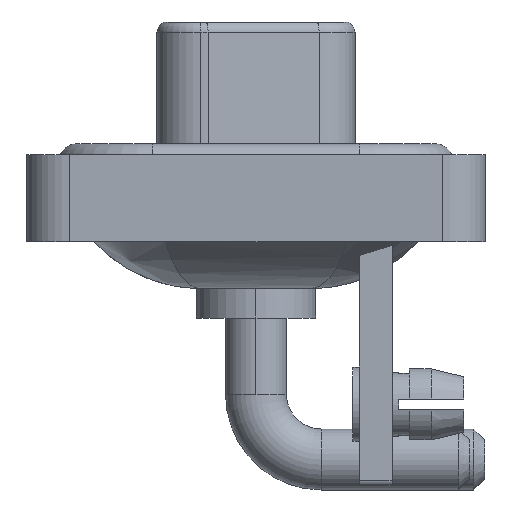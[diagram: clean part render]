
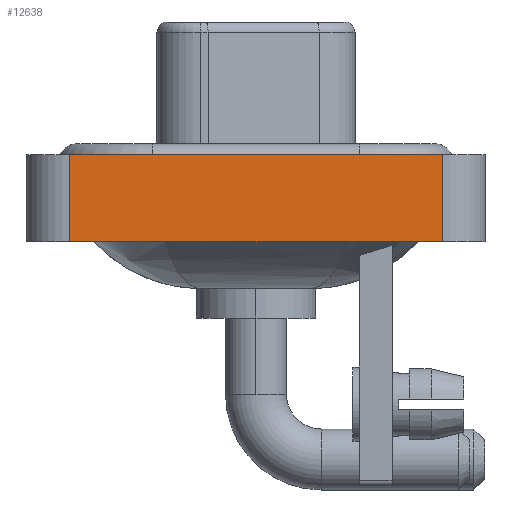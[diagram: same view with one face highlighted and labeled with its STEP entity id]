
A CAD part, left-side view. The second image highlights one B-rep face of the part: STEP entity #12638.
In plain terms, the highlighted planar face has unit normal (-1, 0, 0).
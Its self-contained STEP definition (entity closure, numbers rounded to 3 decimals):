
#395 = ORIENTED_EDGE ( 'NONE', *, *, #15056, .T. ) ;
#424 = DIRECTION ( 'NONE',  ( -1., 0., 0. ) ) ;
#551 = EDGE_CURVE ( 'NONE', #1799, #4549, #3963, .T. ) ;
#833 = CARTESIAN_POINT ( 'NONE',  ( -7.3, -8.55, -3.6 ) ) ;
#1799 = VERTEX_POINT ( 'NONE', #8385 ) ;
#2810 = LINE ( 'NONE', #7864, #3487 ) ;
#3487 = VECTOR ( 'NONE', #6222, 1000. ) ;
#3963 = LINE ( 'NONE', #5728, #11612 ) ;
#4293 = CARTESIAN_POINT ( 'NONE',  ( -7.3, -8.55, 0.4 ) ) ;
#4380 = ORIENTED_EDGE ( 'NONE', *, *, #19439, .T. ) ;
#4383 = VERTEX_POINT ( 'NONE', #833 ) ;
#4549 = VERTEX_POINT ( 'NONE', #11537 ) ;
#4615 = ORIENTED_EDGE ( 'NONE', *, *, #5329, .F. ) ;
#5329 = EDGE_CURVE ( 'NONE', #4549, #21401, #7590, .T. ) ;
#5728 = CARTESIAN_POINT ( 'NONE',  ( -7.3, 8.55, -3.6 ) ) ;
#5864 = DIRECTION ( 'NONE',  ( 0., -1., 0. ) ) ;
#6222 = DIRECTION ( 'NONE',  ( 0., 0., 1. ) ) ;
#7126 = DIRECTION ( 'NONE',  ( 0., 0., 1. ) ) ;
#7590 = LINE ( 'NONE', #4293, #11551 ) ;
#7609 = ORIENTED_EDGE ( 'NONE', *, *, #551, .F. ) ;
#7864 = CARTESIAN_POINT ( 'NONE',  ( -7.3, -8.55, -3.6 ) ) ;
#8385 = CARTESIAN_POINT ( 'NONE',  ( -7.3, 8.55, -3.6 ) ) ;
#9410 = CARTESIAN_POINT ( 'NONE',  ( -7.3, -8.55, 0.4 ) ) ;
#10399 = FACE_OUTER_BOUND ( 'NONE', #15369, .T. ) ;
#10865 = LINE ( 'NONE', #14273, #20759 ) ;
#11537 = CARTESIAN_POINT ( 'NONE',  ( -7.3, 8.55, 0.4 ) ) ;
#11551 = VECTOR ( 'NONE', #12483, 1000. ) ;
#11612 = VECTOR ( 'NONE', #16824, 1000. ) ;
#12483 = DIRECTION ( 'NONE',  ( 0., -1., 0. ) ) ;
#12638 = ADVANCED_FACE ( 'NONE', ( #10399 ), #13670, .T. ) ;
#13442 = AXIS2_PLACEMENT_3D ( 'NONE', #17101, #424, #7126 ) ;
#13670 = PLANE ( 'NONE',  #13442 ) ;
#14273 = CARTESIAN_POINT ( 'NONE',  ( -7.3, -8.55, -3.6 ) ) ;
#15056 = EDGE_CURVE ( 'NONE', #1799, #4383, #10865, .T. ) ;
#15369 = EDGE_LOOP ( 'NONE', ( #4380, #4615, #7609, #395 ) ) ;
#16824 = DIRECTION ( 'NONE',  ( 0., 0., 1. ) ) ;
#17101 = CARTESIAN_POINT ( 'NONE',  ( -7.3, -8.55, -3.6 ) ) ;
#19439 = EDGE_CURVE ( 'NONE', #4383, #21401, #2810, .T. ) ;
#20759 = VECTOR ( 'NONE', #5864, 1000. ) ;
#21401 = VERTEX_POINT ( 'NONE', #9410 ) ;
